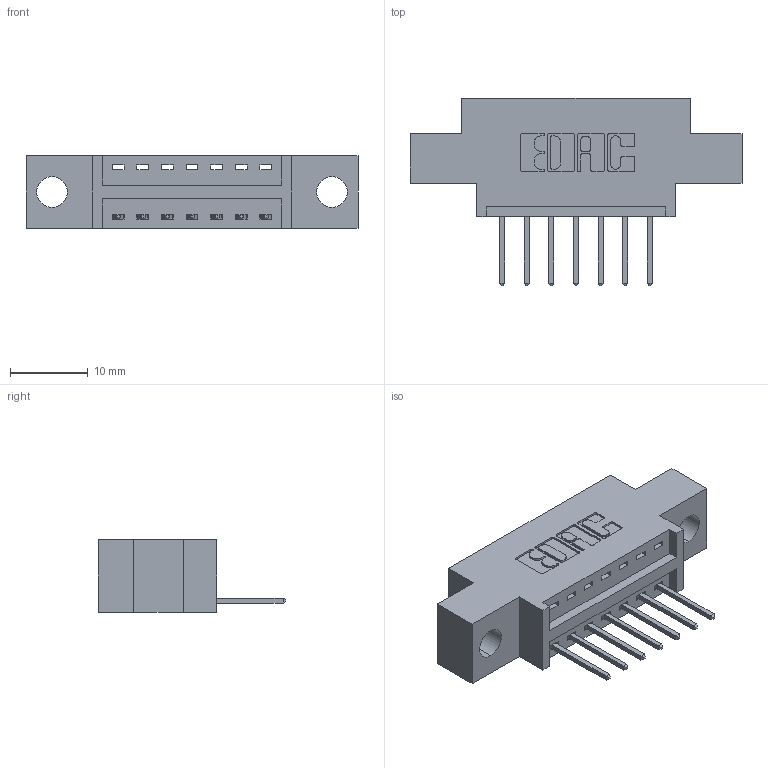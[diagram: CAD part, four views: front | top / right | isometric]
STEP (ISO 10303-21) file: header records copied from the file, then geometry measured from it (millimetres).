
FILE_DESCRIPTION (( 'STEP AP203' ), '1' );
FILE_NAME ('346-007-526-604.STEP', '2022-05-04T19:56:10', ( '' ), ( '' ), 'SwSTEP 2.0', 'SolidWorks 2020', '' );
FILE_SCHEMA (( 'CONFIG_CONTROL_DESIGN' ));
Length unit declared in the file: inch
Products named in the file (3): 346 Part_0.170 Offset - 0.156 Dia-TH; 346-007-526-604; 345-292-001_345-293-126
Assembly tree (8 placements, depth 2):
  346-007-526-604
    346 Part_0.170 Offset - 0.156 Dia-TH
    345-292-001_345-293-126  x7
Bounding box: 42.8 x 24.13 x 9.4 mm (x, y, z)
Volume: 3589.5 mm3; surface area: 4099.5 mm2
Topology: 8 solids, 8 shells, 546 faces, 1609 edges, 1062 vertices
Faces by surface type: plane 374, cylinder 172
Entity records: 9625 total; most frequent: CARTESIAN_POINT 1671, ORIENTED_EDGE 1610, DIRECTION 1515, EDGE_CURVE 805, VECTOR 645, LINE 645, VERTEX_POINT 534, AXIS2_PLACEMENT_3D 435
